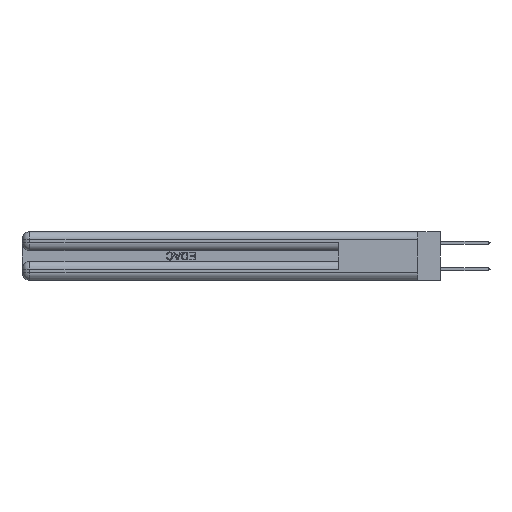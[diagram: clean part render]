
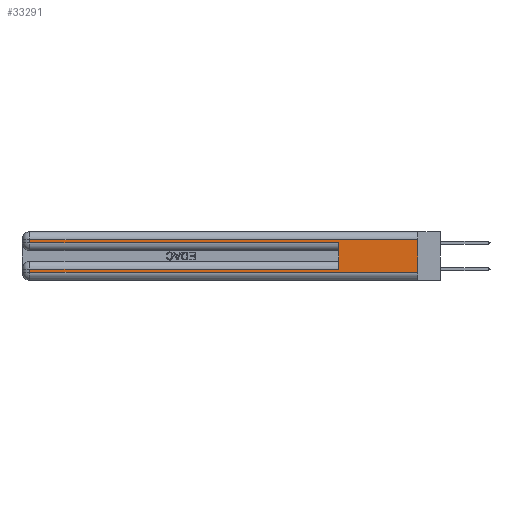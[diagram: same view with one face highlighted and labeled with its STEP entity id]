
A CAD part, left-side view. The second image highlights one B-rep face of the part: STEP entity #33291.
In plain terms, the highlighted planar face has unit normal (-1, 0, 0).
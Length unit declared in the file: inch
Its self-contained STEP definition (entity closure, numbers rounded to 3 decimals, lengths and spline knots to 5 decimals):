
#191 = VECTOR ( 'NONE', #24415, 39.37008 ) ;
#796 = LINE ( 'NONE', #41750, #21413 ) ;
#1580 = DIRECTION ( 'NONE',  ( 0., 0., -1. ) ) ;
#2317 = ORIENTED_EDGE ( 'NONE', *, *, #26430, .T. ) ;
#2432 = EDGE_CURVE ( 'NONE', #18640, #34634, #44290, .T. ) ;
#3638 = CARTESIAN_POINT ( 'NONE',  ( 0., 2.94, 0.085 ) ) ;
#4700 = CARTESIAN_POINT ( 'NONE',  ( 0., 0., 0.06 ) ) ;
#6111 = ORIENTED_EDGE ( 'NONE', *, *, #44334, .T. ) ;
#6967 = VECTOR ( 'NONE', #10223, 39.37008 ) ;
#7001 = ORIENTED_EDGE ( 'NONE', *, *, #22750, .F. ) ;
#8715 = CARTESIAN_POINT ( 'NONE',  ( 0., 2.94, 0.285 ) ) ;
#9143 = CARTESIAN_POINT ( 'NONE',  ( 0., 0., 0.37 ) ) ;
#9651 = VECTOR ( 'NONE', #30404, 39.37008 ) ;
#10223 = DIRECTION ( 'NONE',  ( 0., 1., 0. ) ) ;
#11579 = CARTESIAN_POINT ( 'NONE',  ( 0., 2.94, 0.37 ) ) ;
#12168 = DIRECTION ( 'NONE',  ( 1., 0., 0. ) ) ;
#12255 = LINE ( 'NONE', #11579, #42642 ) ;
#12325 = CARTESIAN_POINT ( 'NONE',  ( 0., 0., 0.37 ) ) ;
#13033 = LINE ( 'NONE', #26898, #9651 ) ;
#13434 = ORIENTED_EDGE ( 'NONE', *, *, #39871, .T. ) ;
#13832 = CARTESIAN_POINT ( 'NONE',  ( 0., 0., 0.085 ) ) ;
#14193 = EDGE_CURVE ( 'NONE', #16653, #41060, #35561, .T. ) ;
#16317 = VECTOR ( 'NONE', #18698, 39.37008 ) ;
#16653 = VERTEX_POINT ( 'NONE', #34755 ) ;
#18640 = VERTEX_POINT ( 'NONE', #44590 ) ;
#18698 = DIRECTION ( 'NONE',  ( 0., -1., 0. ) ) ;
#18782 = LINE ( 'NONE', #9143, #40883 ) ;
#19022 = ORIENTED_EDGE ( 'NONE', *, *, #25014, .F. ) ;
#20807 = ORIENTED_EDGE ( 'NONE', *, *, #29463, .T. ) ;
#21413 = VECTOR ( 'NONE', #38446, 39.37008 ) ;
#22750 = EDGE_CURVE ( 'NONE', #27036, #34829, #796, .T. ) ;
#22798 = PLANE ( 'NONE',  #30565 ) ;
#23689 = ORIENTED_EDGE ( 'NONE', *, *, #2432, .T. ) ;
#24415 = DIRECTION ( 'NONE',  ( 0., 1., 0. ) ) ;
#25014 = EDGE_CURVE ( 'NONE', #18640, #41060, #18782, .T. ) ;
#25134 = LINE ( 'NONE', #33525, #26899 ) ;
#26297 = FACE_OUTER_BOUND ( 'NONE', #46120, .T. ) ;
#26430 = EDGE_CURVE ( 'NONE', #40536, #34829, #13033, .T. ) ;
#26591 = DIRECTION ( 'NONE',  ( 0., 0., -1. ) ) ;
#26652 = CARTESIAN_POINT ( 'NONE',  ( 0., 0.6, 0.285 ) ) ;
#26898 = CARTESIAN_POINT ( 'NONE',  ( 0., 0., 0.285 ) ) ;
#26899 = VECTOR ( 'NONE', #44564, 39.37008 ) ;
#27036 = VERTEX_POINT ( 'NONE', #34579 ) ;
#28188 = ORIENTED_EDGE ( 'NONE', *, *, #14193, .T. ) ;
#29463 = EDGE_CURVE ( 'NONE', #36084, #16653, #25134, .T. ) ;
#30404 = DIRECTION ( 'NONE',  ( 0., -1., 0. ) ) ;
#30565 = AXIS2_PLACEMENT_3D ( 'NONE', #12325, #12168, #26591 ) ;
#33291 = ADVANCED_FACE ( 'NONE', ( #26297 ), #22798, .F. ) ;
#33525 = CARTESIAN_POINT ( 'NONE',  ( 0., 2.94, 0.37 ) ) ;
#34579 = CARTESIAN_POINT ( 'NONE',  ( 0., 0.6, 0.085 ) ) ;
#34634 = VERTEX_POINT ( 'NONE', #41929 ) ;
#34755 = CARTESIAN_POINT ( 'NONE',  ( 0., 2.94, 0.06 ) ) ;
#34829 = VERTEX_POINT ( 'NONE', #26652 ) ;
#35030 = CARTESIAN_POINT ( 'NONE',  ( 0., 0., 0.31 ) ) ;
#35561 = LINE ( 'NONE', #4700, #16317 ) ;
#36084 = VERTEX_POINT ( 'NONE', #3638 ) ;
#38446 = DIRECTION ( 'NONE',  ( 0., 0., 1. ) ) ;
#39871 = EDGE_CURVE ( 'NONE', #34634, #40536, #12255, .T. ) ;
#40536 = VERTEX_POINT ( 'NONE', #8715 ) ;
#40883 = VECTOR ( 'NONE', #1580, 39.37008 ) ;
#41060 = VERTEX_POINT ( 'NONE', #45682 ) ;
#41750 = CARTESIAN_POINT ( 'NONE',  ( 0., 0.6, 0.145 ) ) ;
#41929 = CARTESIAN_POINT ( 'NONE',  ( 0., 2.94, 0.31 ) ) ;
#42642 = VECTOR ( 'NONE', #43822, 39.37008 ) ;
#43822 = DIRECTION ( 'NONE',  ( 0., 0., -1. ) ) ;
#44290 = LINE ( 'NONE', #35030, #191 ) ;
#44334 = EDGE_CURVE ( 'NONE', #27036, #36084, #46027, .T. ) ;
#44564 = DIRECTION ( 'NONE',  ( 0., 0., -1. ) ) ;
#44590 = CARTESIAN_POINT ( 'NONE',  ( 0., 0., 0.31 ) ) ;
#45682 = CARTESIAN_POINT ( 'NONE',  ( 0., 0., 0.06 ) ) ;
#46027 = LINE ( 'NONE', #13832, #6967 ) ;
#46120 = EDGE_LOOP ( 'NONE', ( #19022, #23689, #13434, #2317, #7001, #6111, #20807, #28188 ) ) ;
